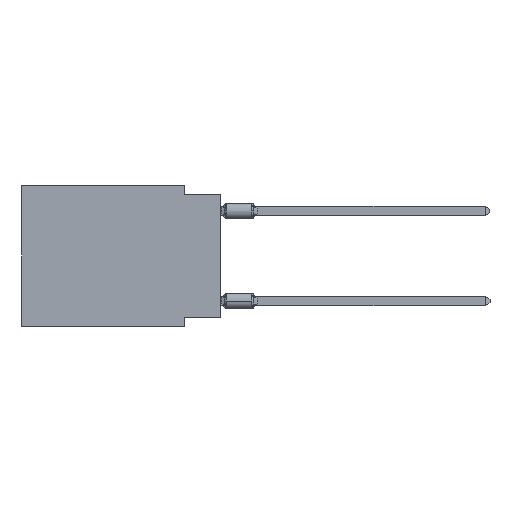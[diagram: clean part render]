
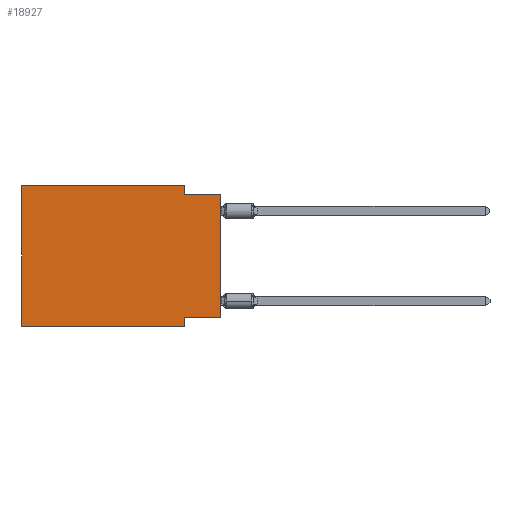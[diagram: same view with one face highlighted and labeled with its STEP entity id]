
A CAD part, left-side view. The second image highlights one B-rep face of the part: STEP entity #18927.
In plain terms, the highlighted planar face has unit normal (-1, 0, 0).
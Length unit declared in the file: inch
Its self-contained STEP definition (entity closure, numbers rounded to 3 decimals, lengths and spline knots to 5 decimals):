
#356 = LINE ( 'NONE', #10306, #20835 ) ;
#500 = DIRECTION ( 'NONE',  ( 0., -1., 0. ) ) ;
#661 = CARTESIAN_POINT ( 'NONE',  ( 0., 0., -0.025 ) ) ;
#1336 = EDGE_CURVE ( 'NONE', #6517, #5334, #7677, .T. ) ;
#2121 = LINE ( 'NONE', #18585, #19096 ) ;
#2377 = CARTESIAN_POINT ( 'NONE',  ( 0., 0., 0. ) ) ;
#2619 = AXIS2_PLACEMENT_3D ( 'NONE', #9577, #14327, #20916 ) ;
#2628 = VECTOR ( 'NONE', #19395, 39.37008 ) ;
#2969 = FACE_OUTER_BOUND ( 'NONE', #18675, .T. ) ;
#2975 = ORIENTED_EDGE ( 'NONE', *, *, #5642, .T. ) ;
#3629 = VERTEX_POINT ( 'NONE', #20057 ) ;
#3885 = CARTESIAN_POINT ( 'NONE',  ( 0., 0.1, 0. ) ) ;
#4580 = LINE ( 'NONE', #5746, #2628 ) ;
#4606 = VECTOR ( 'NONE', #15347, 39.37008 ) ;
#5010 = VECTOR ( 'NONE', #9136, 39.37008 ) ;
#5334 = VERTEX_POINT ( 'NONE', #661 ) ;
#5469 = ORIENTED_EDGE ( 'NONE', *, *, #13330, .F. ) ;
#5514 = CARTESIAN_POINT ( 'NONE',  ( 0., 0.55, -0.39 ) ) ;
#5642 = EDGE_CURVE ( 'NONE', #18961, #16434, #10379, .T. ) ;
#5746 = CARTESIAN_POINT ( 'NONE',  ( 0., 0.1, -0.39 ) ) ;
#6402 = VECTOR ( 'NONE', #500, 39.37008 ) ;
#6517 = VERTEX_POINT ( 'NONE', #10613 ) ;
#6791 = ORIENTED_EDGE ( 'NONE', *, *, #7224, .F. ) ;
#6902 = VECTOR ( 'NONE', #15583, 39.37008 ) ;
#7224 = EDGE_CURVE ( 'NONE', #17824, #3629, #20410, .T. ) ;
#7677 = LINE ( 'NONE', #2377, #6902 ) ;
#7830 = VERTEX_POINT ( 'NONE', #16794 ) ;
#8042 = ORIENTED_EDGE ( 'NONE', *, *, #16156, .F. ) ;
#8292 = CARTESIAN_POINT ( 'NONE',  ( 0., 0.55, 0. ) ) ;
#9136 = DIRECTION ( 'NONE',  ( 0., 0., 1. ) ) ;
#9292 = VERTEX_POINT ( 'NONE', #12477 ) ;
#9539 = CARTESIAN_POINT ( 'NONE',  ( 0., 0.1, -0.39 ) ) ;
#9577 = CARTESIAN_POINT ( 'NONE',  ( 0., 0.55, 0. ) ) ;
#10289 = CARTESIAN_POINT ( 'NONE',  ( 0., 0.1, 0. ) ) ;
#10306 = CARTESIAN_POINT ( 'NONE',  ( 0., 0., -0.365 ) ) ;
#10379 = LINE ( 'NONE', #5514, #10758 ) ;
#10613 = CARTESIAN_POINT ( 'NONE',  ( 0., 0., -0.365 ) ) ;
#10754 = LINE ( 'NONE', #18787, #5010 ) ;
#10758 = VECTOR ( 'NONE', #15362, 39.37008 ) ;
#12477 = CARTESIAN_POINT ( 'NONE',  ( 0., 0.55, 0. ) ) ;
#13223 = ORIENTED_EDGE ( 'NONE', *, *, #1336, .T. ) ;
#13330 = EDGE_CURVE ( 'NONE', #3629, #5334, #2121, .T. ) ;
#13390 = DIRECTION ( 'NONE',  ( 0., -1., 0. ) ) ;
#14327 = DIRECTION ( 'NONE',  ( 1., 0., 0. ) ) ;
#14420 = ORIENTED_EDGE ( 'NONE', *, *, #18669, .F. ) ;
#14784 = ORIENTED_EDGE ( 'NONE', *, *, #17647, .F. ) ;
#15347 = DIRECTION ( 'NONE',  ( 0., 0., -1. ) ) ;
#15362 = DIRECTION ( 'NONE',  ( 0., -1., 0. ) ) ;
#15578 = ORIENTED_EDGE ( 'NONE', *, *, #21298, .F. ) ;
#15583 = DIRECTION ( 'NONE',  ( 0., 0., 1. ) ) ;
#16156 = EDGE_CURVE ( 'NONE', #6517, #7830, #356, .T. ) ;
#16284 = PLANE ( 'NONE',  #2619 ) ;
#16434 = VERTEX_POINT ( 'NONE', #9539 ) ;
#16794 = CARTESIAN_POINT ( 'NONE',  ( 0., 0.1, -0.365 ) ) ;
#17647 = EDGE_CURVE ( 'NONE', #18961, #9292, #10754, .T. ) ;
#17706 = CARTESIAN_POINT ( 'NONE',  ( 0., 0.55, -0.39 ) ) ;
#17824 = VERTEX_POINT ( 'NONE', #10289 ) ;
#18585 = CARTESIAN_POINT ( 'NONE',  ( 0., 0., -0.025 ) ) ;
#18669 = EDGE_CURVE ( 'NONE', #9292, #17824, #19865, .T. ) ;
#18675 = EDGE_LOOP ( 'NONE', ( #13223, #5469, #6791, #14420, #14784, #2975, #15578, #8042 ) ) ;
#18787 = CARTESIAN_POINT ( 'NONE',  ( 0., 0.55, 0. ) ) ;
#18927 = ADVANCED_FACE ( 'NONE', ( #2969 ), #16284, .F. ) ;
#18961 = VERTEX_POINT ( 'NONE', #17706 ) ;
#19096 = VECTOR ( 'NONE', #13390, 39.37008 ) ;
#19395 = DIRECTION ( 'NONE',  ( 0., 0., -1. ) ) ;
#19865 = LINE ( 'NONE', #8292, #6402 ) ;
#20057 = CARTESIAN_POINT ( 'NONE',  ( 0., 0.1, -0.025 ) ) ;
#20250 = DIRECTION ( 'NONE',  ( 0., 1., 0. ) ) ;
#20410 = LINE ( 'NONE', #3885, #4606 ) ;
#20835 = VECTOR ( 'NONE', #20250, 39.37008 ) ;
#20916 = DIRECTION ( 'NONE',  ( 0., 0., -1. ) ) ;
#21298 = EDGE_CURVE ( 'NONE', #7830, #16434, #4580, .T. ) ;
